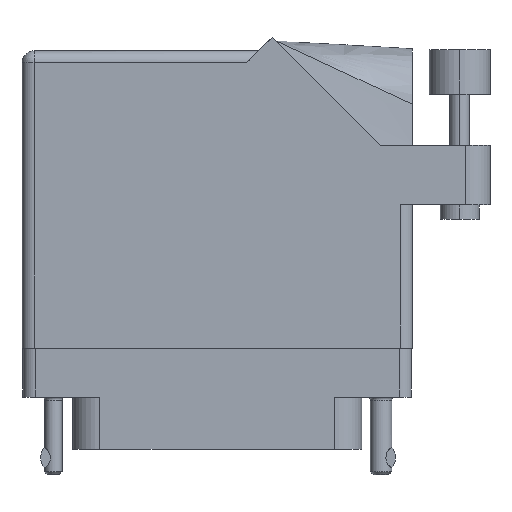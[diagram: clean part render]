
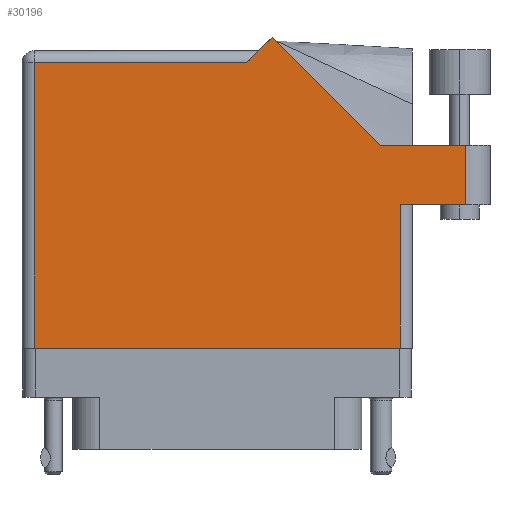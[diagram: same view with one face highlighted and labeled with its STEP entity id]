
A CAD part, front view. The second image highlights one B-rep face of the part: STEP entity #30196.
In plain terms, the highlighted face is planar.
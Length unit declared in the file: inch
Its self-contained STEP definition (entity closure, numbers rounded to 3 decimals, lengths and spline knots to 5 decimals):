
#553 = EDGE_CURVE ( 'NONE', #15762, #39507, #15314, .T. ) ;
#827 = EDGE_LOOP ( 'NONE', ( #39454, #3762, #8792, #39504, #5543, #22702, #17782, #41797, #47588 ) ) ;
#885 = DIRECTION ( 'NONE',  ( -0.707, 0.707, 0. ) ) ;
#983 = VECTOR ( 'NONE', #40013, 39.37008 ) ;
#1232 = CARTESIAN_POINT ( 'NONE',  ( 0.83942, 0.944, 0.455 ) ) ;
#3762 = ORIENTED_EDGE ( 'NONE', *, *, #47944, .T. ) ;
#4761 = EDGE_CURVE ( 'NONE', #48106, #20066, #41092, .T. ) ;
#5051 = EDGE_CURVE ( 'NONE', #24160, #48106, #30826, .T. ) ;
#5471 = VECTOR ( 'NONE', #16604, 39.37008 ) ;
#5543 = ORIENTED_EDGE ( 'NONE', *, *, #28642, .T. ) ;
#6367 = LINE ( 'NONE', #47511, #983 ) ;
#6455 = EDGE_CURVE ( 'NONE', #15893, #7682, #42668, .T. ) ;
#7350 = EDGE_CURVE ( 'NONE', #7682, #24633, #6367, .T. ) ;
#7682 = VERTEX_POINT ( 'NONE', #14091 ) ;
#8146 = PLANE ( 'NONE',  #12213 ) ;
#8792 = ORIENTED_EDGE ( 'NONE', *, *, #5051, .T. ) ;
#9516 = VECTOR ( 'NONE', #33560, 39.37008 ) ;
#9898 = DIRECTION ( 'NONE',  ( -1., 0., 0. ) ) ;
#11448 = EDGE_CURVE ( 'NONE', #39507, #12810, #42933, .T. ) ;
#12213 = AXIS2_PLACEMENT_3D ( 'NONE', #12604, #19691, #20019 ) ;
#12493 = CARTESIAN_POINT ( 'NONE',  ( -0.943, -0.1, 0.455 ) ) ;
#12604 = CARTESIAN_POINT ( 'NONE',  ( -1.005, 1.43, 0.455 ) ) ;
#12732 = VECTOR ( 'NONE', #48883, 39.37008 ) ;
#12810 = VERTEX_POINT ( 'NONE', #23460 ) ;
#13047 = VECTOR ( 'NONE', #9898, 39.37008 ) ;
#13487 = CARTESIAN_POINT ( 'NONE',  ( 1.28, 0.637, 0.455 ) ) ;
#14091 = CARTESIAN_POINT ( 'NONE',  ( 0.943, 0.637, 0.455 ) ) ;
#15314 = LINE ( 'NONE', #31067, #36100 ) ;
#15561 = CARTESIAN_POINT ( 'NONE',  ( 0.15, 1.368, 0.455 ) ) ;
#15762 = VERTEX_POINT ( 'NONE', #15561 ) ;
#15893 = VERTEX_POINT ( 'NONE', #20811 ) ;
#15927 = CARTESIAN_POINT ( 'NONE',  ( 0.212, 1.43, 0.455 ) ) ;
#16604 = DIRECTION ( 'NONE',  ( 0., -1., 0. ) ) ;
#16916 = CARTESIAN_POINT ( 'NONE',  ( 1.28, 0.944, 0.455 ) ) ;
#17782 = ORIENTED_EDGE ( 'NONE', *, *, #11448, .T. ) ;
#18114 = CARTESIAN_POINT ( 'NONE',  ( -1.005, -0.1, 0.455 ) ) ;
#18424 = VECTOR ( 'NONE', #885, 39.37008 ) ;
#19691 = DIRECTION ( 'NONE',  ( 0., 0., -1. ) ) ;
#19756 = DIRECTION ( 'NONE',  ( -1., 0., 0. ) ) ;
#20019 = DIRECTION ( 'NONE',  ( -1., 0., 0. ) ) ;
#20066 = VERTEX_POINT ( 'NONE', #20831 ) ;
#20811 = CARTESIAN_POINT ( 'NONE',  ( 0.943, -0.1, 0.455 ) ) ;
#20831 = CARTESIAN_POINT ( 'NONE',  ( 0.28271, 1.50071, 0.455 ) ) ;
#22702 = ORIENTED_EDGE ( 'NONE', *, *, #553, .T. ) ;
#23460 = CARTESIAN_POINT ( 'NONE',  ( -0.943, -0.1, 0.455 ) ) ;
#23667 = DIRECTION ( 'NONE',  ( 0., 1., 0. ) ) ;
#24160 = VERTEX_POINT ( 'NONE', #16916 ) ;
#24633 = VERTEX_POINT ( 'NONE', #13487 ) ;
#26852 = CARTESIAN_POINT ( 'NONE',  ( 0.943, 0.637, 0.455 ) ) ;
#28347 = EDGE_CURVE ( 'NONE', #12810, #15893, #48218, .T. ) ;
#28642 = EDGE_CURVE ( 'NONE', #20066, #15762, #42789, .T. ) ;
#28962 = VECTOR ( 'NONE', #23667, 39.37008 ) ;
#30196 = ADVANCED_FACE ( 'NONE', ( #38476 ), #8146, .F. ) ;
#30826 = LINE ( 'NONE', #32601, #13047 ) ;
#31067 = CARTESIAN_POINT ( 'NONE',  ( -1.005, 1.368, 0.455 ) ) ;
#31341 = DIRECTION ( 'NONE',  ( -0.707, -0.707, 0. ) ) ;
#32601 = CARTESIAN_POINT ( 'NONE',  ( 1.405, 0.944, 0.455 ) ) ;
#32942 = LINE ( 'NONE', #48713, #12732 ) ;
#33235 = VECTOR ( 'NONE', #31341, 39.37008 ) ;
#33560 = DIRECTION ( 'NONE',  ( 1., 0., 0. ) ) ;
#34317 = CARTESIAN_POINT ( 'NONE',  ( 0.83942, 0.944, 0.455 ) ) ;
#36100 = VECTOR ( 'NONE', #19756, 39.37008 ) ;
#38476 = FACE_OUTER_BOUND ( 'NONE', #827, .T. ) ;
#39454 = ORIENTED_EDGE ( 'NONE', *, *, #7350, .T. ) ;
#39504 = ORIENTED_EDGE ( 'NONE', *, *, #4761, .T. ) ;
#39507 = VERTEX_POINT ( 'NONE', #48364 ) ;
#40013 = DIRECTION ( 'NONE',  ( 1., 0., 0. ) ) ;
#41092 = LINE ( 'NONE', #1232, #18424 ) ;
#41797 = ORIENTED_EDGE ( 'NONE', *, *, #28347, .T. ) ;
#42668 = LINE ( 'NONE', #26852, #28962 ) ;
#42789 = LINE ( 'NONE', #15927, #33235 ) ;
#42933 = LINE ( 'NONE', #12493, #5471 ) ;
#47511 = CARTESIAN_POINT ( 'NONE',  ( 1.005, 0.637, 0.455 ) ) ;
#47588 = ORIENTED_EDGE ( 'NONE', *, *, #6455, .T. ) ;
#47944 = EDGE_CURVE ( 'NONE', #24633, #24160, #32942, .T. ) ;
#48106 = VERTEX_POINT ( 'NONE', #34317 ) ;
#48218 = LINE ( 'NONE', #18114, #9516 ) ;
#48364 = CARTESIAN_POINT ( 'NONE',  ( -0.943, 1.368, 0.455 ) ) ;
#48713 = CARTESIAN_POINT ( 'NONE',  ( 1.28, 0.944, 0.455 ) ) ;
#48883 = DIRECTION ( 'NONE',  ( 0., 1., 0. ) ) ;
